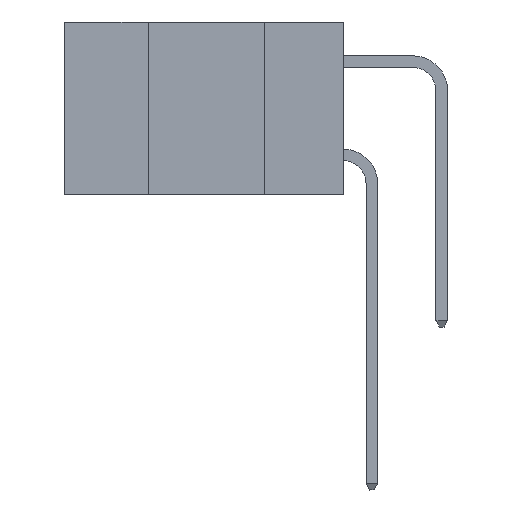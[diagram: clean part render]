
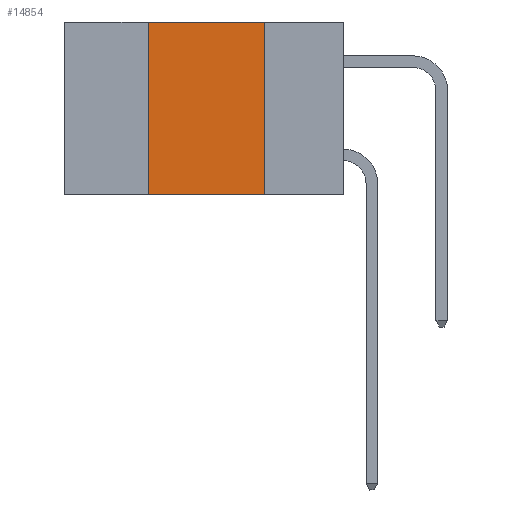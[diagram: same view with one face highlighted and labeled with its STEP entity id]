
A CAD part, left-side view. The second image highlights one B-rep face of the part: STEP entity #14854.
In plain terms, the highlighted planar face has unit normal (-1, 0, 0).
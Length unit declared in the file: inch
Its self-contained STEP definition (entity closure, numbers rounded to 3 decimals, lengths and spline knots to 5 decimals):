
#502 = CARTESIAN_POINT ( 'NONE',  ( 0., 0.17, 0. ) ) ;
#1717 = VECTOR ( 'NONE', #4212, 39.37008 ) ;
#1817 = VERTEX_POINT ( 'NONE', #502 ) ;
#2303 = DIRECTION ( 'NONE',  ( 1., 0., 0. ) ) ;
#2341 = LINE ( 'NONE', #17328, #1717 ) ;
#2392 = LINE ( 'NONE', #18398, #5671 ) ;
#2519 = CARTESIAN_POINT ( 'NONE',  ( 0., 0.42, -0.37 ) ) ;
#2844 = CARTESIAN_POINT ( 'NONE',  ( 0., 0.6, 0. ) ) ;
#3055 = EDGE_LOOP ( 'NONE', ( #21920, #12076, #11089, #22222 ) ) ;
#3671 = CARTESIAN_POINT ( 'NONE',  ( 0., 0.42, 0. ) ) ;
#4212 = DIRECTION ( 'NONE',  ( 0., 0., -1. ) ) ;
#4469 = LINE ( 'NONE', #2844, #13952 ) ;
#5671 = VECTOR ( 'NONE', #7249, 39.37008 ) ;
#6497 = VERTEX_POINT ( 'NONE', #2519 ) ;
#6611 = DIRECTION ( 'NONE',  ( 0., -1., 0. ) ) ;
#6966 = VECTOR ( 'NONE', #7423, 39.37008 ) ;
#7249 = DIRECTION ( 'NONE',  ( 0., 0., 1. ) ) ;
#7423 = DIRECTION ( 'NONE',  ( 0., -1., 0. ) ) ;
#8010 = FACE_OUTER_BOUND ( 'NONE', #3055, .T. ) ;
#9835 = EDGE_CURVE ( 'NONE', #6497, #13667, #16302, .T. ) ;
#11089 = ORIENTED_EDGE ( 'NONE', *, *, #12367, .F. ) ;
#12076 = ORIENTED_EDGE ( 'NONE', *, *, #13644, .F. ) ;
#12367 = EDGE_CURVE ( 'NONE', #6497, #15935, #2392, .T. ) ;
#13644 = EDGE_CURVE ( 'NONE', #15935, #1817, #4469, .T. ) ;
#13652 = CARTESIAN_POINT ( 'NONE',  ( 0., 0.6, 0. ) ) ;
#13667 = VERTEX_POINT ( 'NONE', #14187 ) ;
#13952 = VECTOR ( 'NONE', #6611, 39.37008 ) ;
#14187 = CARTESIAN_POINT ( 'NONE',  ( 0., 0.17, -0.37 ) ) ;
#14854 = ADVANCED_FACE ( 'NONE', ( #8010 ), #20971, .F. ) ;
#14861 = EDGE_CURVE ( 'NONE', #1817, #13667, #2341, .T. ) ;
#15470 = DIRECTION ( 'NONE',  ( 0., 0., -1. ) ) ;
#15935 = VERTEX_POINT ( 'NONE', #3671 ) ;
#16302 = LINE ( 'NONE', #18565, #6966 ) ;
#17328 = CARTESIAN_POINT ( 'NONE',  ( 0., 0.17, -0.37 ) ) ;
#18398 = CARTESIAN_POINT ( 'NONE',  ( 0., 0.42, -0.37 ) ) ;
#18565 = CARTESIAN_POINT ( 'NONE',  ( 0., 0.6, -0.37 ) ) ;
#20971 = PLANE ( 'NONE',  #21063 ) ;
#21063 = AXIS2_PLACEMENT_3D ( 'NONE', #13652, #2303, #15470 ) ;
#21920 = ORIENTED_EDGE ( 'NONE', *, *, #14861, .F. ) ;
#22222 = ORIENTED_EDGE ( 'NONE', *, *, #9835, .T. ) ;
